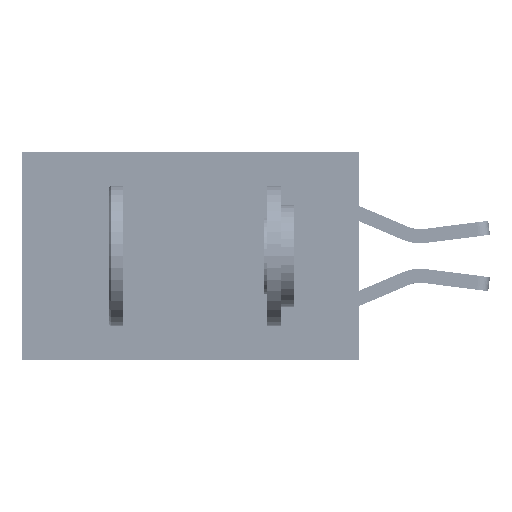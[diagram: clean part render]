
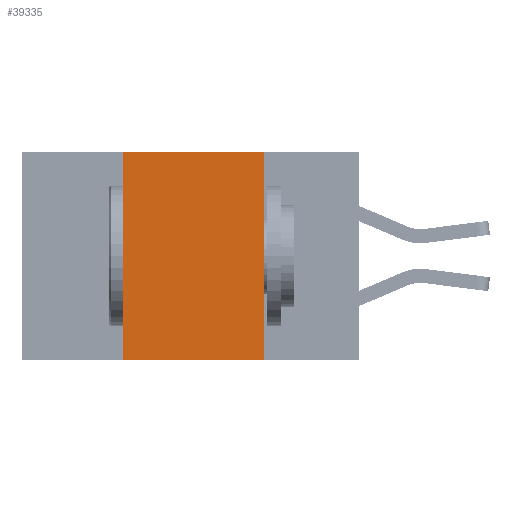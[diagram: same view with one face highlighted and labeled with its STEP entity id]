
A CAD part, left-side view. The second image highlights one B-rep face of the part: STEP entity #39335.
In plain terms, the highlighted planar face has unit normal (-1, 0, 0).
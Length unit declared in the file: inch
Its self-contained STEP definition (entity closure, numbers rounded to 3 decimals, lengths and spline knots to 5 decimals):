
#946 = CARTESIAN_POINT ( 'NONE',  ( 0., 0.42, -0.37 ) ) ;
#1870 = VERTEX_POINT ( 'NONE', #35275 ) ;
#2975 = ORIENTED_EDGE ( 'NONE', *, *, #6268, .F. ) ;
#5053 = ORIENTED_EDGE ( 'NONE', *, *, #35180, .T. ) ;
#6268 = EDGE_CURVE ( 'NONE', #30075, #20600, #8630, .T. ) ;
#6601 = VECTOR ( 'NONE', #16694, 39.37008 ) ;
#7634 = EDGE_CURVE ( 'NONE', #1870, #35161, #32234, .T. ) ;
#7807 = CARTESIAN_POINT ( 'NONE',  ( 0., 0.6, 0. ) ) ;
#8630 = LINE ( 'NONE', #41750, #40871 ) ;
#9626 = LINE ( 'NONE', #19023, #17221 ) ;
#11375 = EDGE_LOOP ( 'NONE', ( #19228, #27757, #2975, #5053 ) ) ;
#13442 = CARTESIAN_POINT ( 'NONE',  ( 0., 0.6, 0. ) ) ;
#13831 = FACE_OUTER_BOUND ( 'NONE', #11375, .T. ) ;
#14355 = DIRECTION ( 'NONE',  ( 0., 0., -1. ) ) ;
#15113 = VECTOR ( 'NONE', #26650, 39.37008 ) ;
#16126 = CARTESIAN_POINT ( 'NONE',  ( 0., 0.42, 0. ) ) ;
#16236 = CARTESIAN_POINT ( 'NONE',  ( 0., 0.17, 0. ) ) ;
#16694 = DIRECTION ( 'NONE',  ( 0., -1., 0. ) ) ;
#17221 = VECTOR ( 'NONE', #35056, 39.37008 ) ;
#19023 = CARTESIAN_POINT ( 'NONE',  ( 0., 0.6, -0.37 ) ) ;
#19228 = ORIENTED_EDGE ( 'NONE', *, *, #7634, .F. ) ;
#20600 = VERTEX_POINT ( 'NONE', #16126 ) ;
#26650 = DIRECTION ( 'NONE',  ( 0., 0., -1. ) ) ;
#27757 = ORIENTED_EDGE ( 'NONE', *, *, #29233, .F. ) ;
#29233 = EDGE_CURVE ( 'NONE', #20600, #1870, #33371, .T. ) ;
#30075 = VERTEX_POINT ( 'NONE', #946 ) ;
#30413 = PLANE ( 'NONE',  #34721 ) ;
#31832 = CARTESIAN_POINT ( 'NONE',  ( 0., 0.17, -0.37 ) ) ;
#32234 = LINE ( 'NONE', #16236, #15113 ) ;
#33371 = LINE ( 'NONE', #13442, #6601 ) ;
#33632 = DIRECTION ( 'NONE',  ( 1., 0., 0. ) ) ;
#34721 = AXIS2_PLACEMENT_3D ( 'NONE', #7807, #33632, #14355 ) ;
#35056 = DIRECTION ( 'NONE',  ( 0., -1., 0. ) ) ;
#35161 = VERTEX_POINT ( 'NONE', #31832 ) ;
#35180 = EDGE_CURVE ( 'NONE', #30075, #35161, #9626, .T. ) ;
#35275 = CARTESIAN_POINT ( 'NONE',  ( 0., 0.17, 0. ) ) ;
#38565 = DIRECTION ( 'NONE',  ( 0., 0., 1. ) ) ;
#39335 = ADVANCED_FACE ( 'NONE', ( #13831 ), #30413, .F. ) ;
#40871 = VECTOR ( 'NONE', #38565, 39.37008 ) ;
#41750 = CARTESIAN_POINT ( 'NONE',  ( 0., 0.42, 0. ) ) ;
